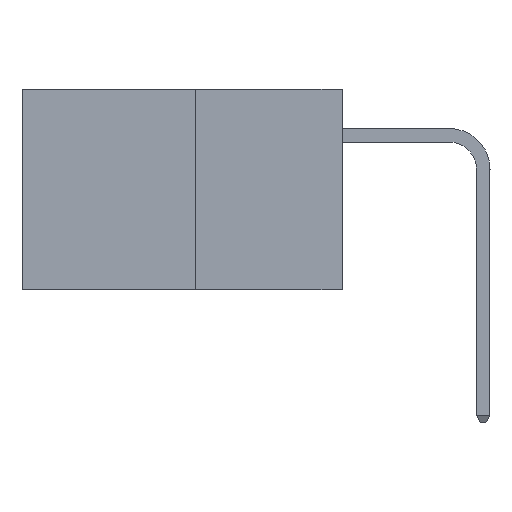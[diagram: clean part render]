
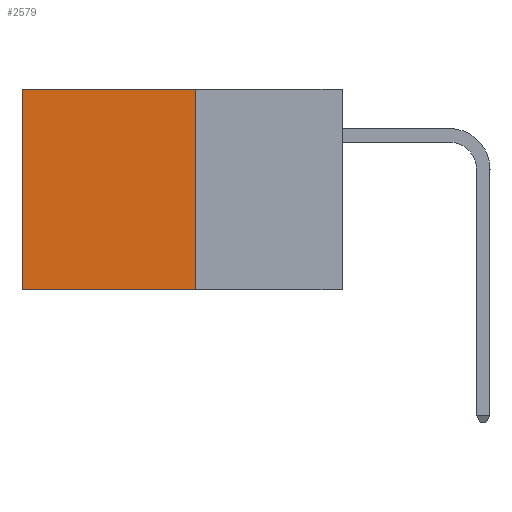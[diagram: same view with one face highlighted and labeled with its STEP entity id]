
A CAD part, left-side view. The second image highlights one B-rep face of the part: STEP entity #2579.
In plain terms, the highlighted planar face has unit normal (-1, 0, 0).
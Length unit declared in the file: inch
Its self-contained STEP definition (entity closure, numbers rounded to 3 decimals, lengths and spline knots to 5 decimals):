
#153 = VERTEX_POINT ( 'NONE', #4241 ) ;
#251 = EDGE_LOOP ( 'NONE', ( #679, #4775, #9790, #7181 ) ) ;
#679 = ORIENTED_EDGE ( 'NONE', *, *, #7125, .T. ) ;
#820 = VECTOR ( 'NONE', #6635, 39.37008 ) ;
#844 = LINE ( 'NONE', #13967, #6822 ) ;
#2579 = ADVANCED_FACE ( 'NONE', ( #6273 ), #10799, .F. ) ;
#4024 = LINE ( 'NONE', #7441, #7326 ) ;
#4050 = AXIS2_PLACEMENT_3D ( 'NONE', #14269, #9047, #10073 ) ;
#4241 = CARTESIAN_POINT ( 'NONE',  ( 0.277, 0.59, 0. ) ) ;
#4275 = VECTOR ( 'NONE', #6943, 39.37008 ) ;
#4291 = EDGE_CURVE ( 'NONE', #6184, #153, #7871, .T. ) ;
#4775 = ORIENTED_EDGE ( 'NONE', *, *, #7908, .F. ) ;
#5290 = DIRECTION ( 'NONE',  ( 0., 0., -1. ) ) ;
#5532 = CARTESIAN_POINT ( 'NONE',  ( 0.277, 0.27, -0.37 ) ) ;
#6134 = VERTEX_POINT ( 'NONE', #13204 ) ;
#6184 = VERTEX_POINT ( 'NONE', #7744 ) ;
#6273 = FACE_OUTER_BOUND ( 'NONE', #251, .T. ) ;
#6386 = DIRECTION ( 'NONE',  ( 0., 0., -1. ) ) ;
#6635 = DIRECTION ( 'NONE',  ( 0., 1., 0. ) ) ;
#6822 = VECTOR ( 'NONE', #6386, 39.37008 ) ;
#6943 = DIRECTION ( 'NONE',  ( 0., 1., 0. ) ) ;
#7008 = CARTESIAN_POINT ( 'NONE',  ( 0.277, 0.27, 0. ) ) ;
#7125 = EDGE_CURVE ( 'NONE', #153, #6134, #844, .T. ) ;
#7181 = ORIENTED_EDGE ( 'NONE', *, *, #4291, .T. ) ;
#7326 = VECTOR ( 'NONE', #5290, 39.37008 ) ;
#7441 = CARTESIAN_POINT ( 'NONE',  ( 0.277, 0.27, -0.37 ) ) ;
#7744 = CARTESIAN_POINT ( 'NONE',  ( 0.277, 0.27, 0. ) ) ;
#7871 = LINE ( 'NONE', #7008, #4275 ) ;
#7908 = EDGE_CURVE ( 'NONE', #11420, #6134, #9741, .T. ) ;
#9047 = DIRECTION ( 'NONE',  ( 1., 0., 0. ) ) ;
#9741 = LINE ( 'NONE', #5532, #820 ) ;
#9790 = ORIENTED_EDGE ( 'NONE', *, *, #12615, .F. ) ;
#10073 = DIRECTION ( 'NONE',  ( 0., 0., -1. ) ) ;
#10799 = PLANE ( 'NONE',  #4050 ) ;
#11420 = VERTEX_POINT ( 'NONE', #13925 ) ;
#12615 = EDGE_CURVE ( 'NONE', #6184, #11420, #4024, .T. ) ;
#13204 = CARTESIAN_POINT ( 'NONE',  ( 0.277, 0.59, -0.37 ) ) ;
#13925 = CARTESIAN_POINT ( 'NONE',  ( 0.277, 0.27, -0.37 ) ) ;
#13967 = CARTESIAN_POINT ( 'NONE',  ( 0.277, 0.59, -0.37 ) ) ;
#14269 = CARTESIAN_POINT ( 'NONE',  ( 0.277, 0.27, -0.37 ) ) ;
